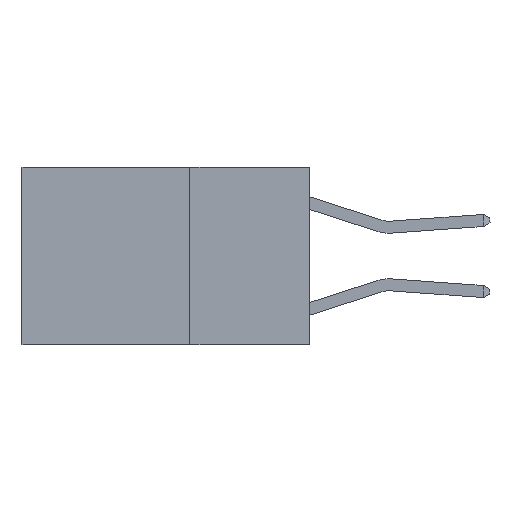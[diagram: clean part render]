
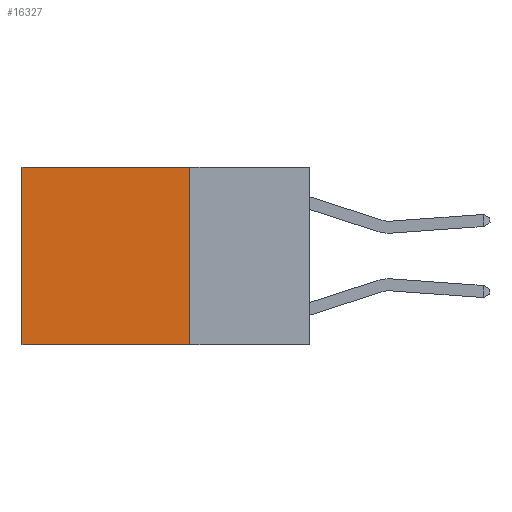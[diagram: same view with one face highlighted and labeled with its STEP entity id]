
A CAD part, left-side view. The second image highlights one B-rep face of the part: STEP entity #16327.
In plain terms, the highlighted planar face has unit normal (-1, 0, 0).
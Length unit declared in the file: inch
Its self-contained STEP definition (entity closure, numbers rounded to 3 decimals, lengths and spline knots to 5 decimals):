
#422 = ORIENTED_EDGE ( 'NONE', *, *, #4918, .T. ) ;
#1788 = EDGE_LOOP ( 'NONE', ( #422, #3277, #11789, #17919 ) ) ;
#2453 = VERTEX_POINT ( 'NONE', #7279 ) ;
#3277 = ORIENTED_EDGE ( 'NONE', *, *, #16700, .F. ) ;
#4067 = CARTESIAN_POINT ( 'NONE',  ( 0.2625, 0.25, -0.37 ) ) ;
#4270 = LINE ( 'NONE', #15866, #8889 ) ;
#4918 = EDGE_CURVE ( 'NONE', #17302, #2453, #12288, .T. ) ;
#6236 = VECTOR ( 'NONE', #18667, 39.37008 ) ;
#7201 = EDGE_CURVE ( 'NONE', #12410, #15671, #4270, .T. ) ;
#7279 = CARTESIAN_POINT ( 'NONE',  ( 0.2625, 0.6, -0.37 ) ) ;
#8889 = VECTOR ( 'NONE', #17815, 39.37008 ) ;
#11789 = ORIENTED_EDGE ( 'NONE', *, *, #7201, .F. ) ;
#12131 = CARTESIAN_POINT ( 'NONE',  ( 0.2625, 0.25, 0. ) ) ;
#12288 = LINE ( 'NONE', #24024, #6236 ) ;
#12410 = VERTEX_POINT ( 'NONE', #14596 ) ;
#12817 = CARTESIAN_POINT ( 'NONE',  ( 0.2625, 0.6, 0. ) ) ;
#13170 = EDGE_CURVE ( 'NONE', #12410, #17302, #24258, .T. ) ;
#13856 = DIRECTION ( 'NONE',  ( 0., 0., -1. ) ) ;
#14017 = VECTOR ( 'NONE', #20859, 39.37008 ) ;
#14321 = CARTESIAN_POINT ( 'NONE',  ( 0.2625, 0.25, -0.37 ) ) ;
#14596 = CARTESIAN_POINT ( 'NONE',  ( 0.2625, 0.25, 0. ) ) ;
#15671 = VERTEX_POINT ( 'NONE', #4067 ) ;
#15751 = FACE_OUTER_BOUND ( 'NONE', #1788, .T. ) ;
#15797 = PLANE ( 'NONE',  #21096 ) ;
#15866 = CARTESIAN_POINT ( 'NONE',  ( 0.2625, 0.25, 0. ) ) ;
#16327 = ADVANCED_FACE ( 'NONE', ( #15751 ), #15797, .F. ) ;
#16700 = EDGE_CURVE ( 'NONE', #15671, #2453, #22244, .T. ) ;
#17002 = CARTESIAN_POINT ( 'NONE',  ( 0.2625, 0.25, 0. ) ) ;
#17157 = VECTOR ( 'NONE', #20077, 39.37008 ) ;
#17302 = VERTEX_POINT ( 'NONE', #12817 ) ;
#17815 = DIRECTION ( 'NONE',  ( 0., 0., -1. ) ) ;
#17919 = ORIENTED_EDGE ( 'NONE', *, *, #13170, .T. ) ;
#18667 = DIRECTION ( 'NONE',  ( 0., 0., -1. ) ) ;
#19657 = DIRECTION ( 'NONE',  ( 1., 0., 0. ) ) ;
#20077 = DIRECTION ( 'NONE',  ( 0., 1., 0. ) ) ;
#20859 = DIRECTION ( 'NONE',  ( 0., 1., 0. ) ) ;
#21096 = AXIS2_PLACEMENT_3D ( 'NONE', #12131, #19657, #13856 ) ;
#22244 = LINE ( 'NONE', #14321, #17157 ) ;
#24024 = CARTESIAN_POINT ( 'NONE',  ( 0.2625, 0.6, 0. ) ) ;
#24258 = LINE ( 'NONE', #17002, #14017 ) ;
